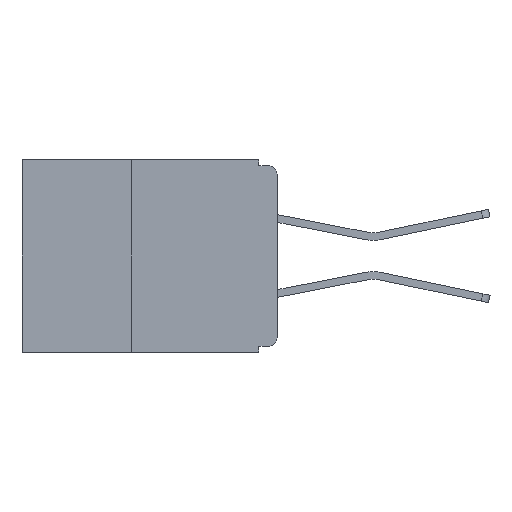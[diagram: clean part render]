
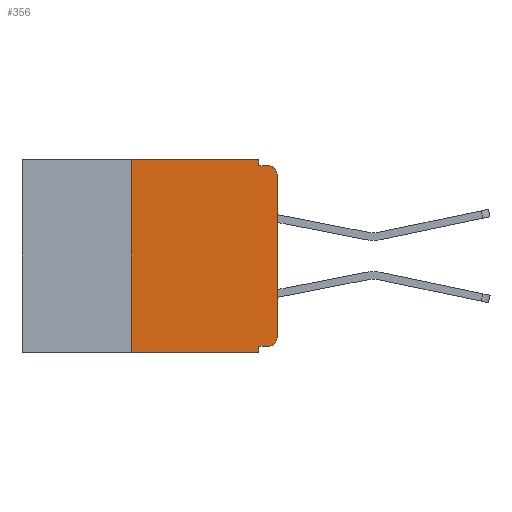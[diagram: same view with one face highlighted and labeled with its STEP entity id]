
A CAD part, left-side view. The second image highlights one B-rep face of the part: STEP entity #356.
In plain terms, the highlighted planar face has unit normal (-1, 0, 0).
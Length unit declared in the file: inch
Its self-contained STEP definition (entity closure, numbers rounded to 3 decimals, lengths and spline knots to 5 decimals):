
#95 = DIRECTION ( 'NONE',  ( 1., 0., 0. ) ) ;
#102 = DIRECTION ( 'NONE',  ( 0., 0., 1. ) ) ;
#113 = LINE ( 'NONE', #15190, #7937 ) ;
#356 = ADVANCED_FACE ( 'NONE', ( #10847 ), #14837, .F. ) ;
#819 = ORIENTED_EDGE ( 'NONE', *, *, #11171, .T. ) ;
#977 = CARTESIAN_POINT ( 'NONE',  ( 0., 0.031, -0.32 ) ) ;
#2271 = VERTEX_POINT ( 'NONE', #977 ) ;
#2440 = ORIENTED_EDGE ( 'NONE', *, *, #7968, .F. ) ;
#2616 = LINE ( 'NONE', #19415, #6744 ) ;
#2695 = CARTESIAN_POINT ( 'NONE',  ( 0., 0.031, -0.33 ) ) ;
#2927 = DIRECTION ( 'NONE',  ( -1., 0., 0. ) ) ;
#2969 = ORIENTED_EDGE ( 'NONE', *, *, #9448, .T. ) ;
#3210 = CARTESIAN_POINT ( 'NONE',  ( 0., 0., -0.025 ) ) ;
#3247 = CARTESIAN_POINT ( 'NONE',  ( 0., 0., -0.01 ) ) ;
#3523 = VECTOR ( 'NONE', #102, 39.37008 ) ;
#3764 = VERTEX_POINT ( 'NONE', #5513 ) ;
#3935 = CARTESIAN_POINT ( 'NONE',  ( 0., 0.015, -0.01 ) ) ;
#3939 = DIRECTION ( 'NONE',  ( 0., -1., 0. ) ) ;
#4456 = VERTEX_POINT ( 'NONE', #14680 ) ;
#4615 = CIRCLE ( 'NONE', #9679, 0.015 ) ;
#4623 = DIRECTION ( 'NONE',  ( 0., 0., -1. ) ) ;
#4911 = ORIENTED_EDGE ( 'NONE', *, *, #19390, .F. ) ;
#5103 = VERTEX_POINT ( 'NONE', #3210 ) ;
#5513 = CARTESIAN_POINT ( 'NONE',  ( 0., 0.25, 0. ) ) ;
#6025 = ORIENTED_EDGE ( 'NONE', *, *, #6124, .F. ) ;
#6053 = LINE ( 'NONE', #13020, #13586 ) ;
#6124 = EDGE_CURVE ( 'NONE', #19385, #2271, #113, .T. ) ;
#6363 = DIRECTION ( 'NONE',  ( 0., -1., 0. ) ) ;
#6632 = VERTEX_POINT ( 'NONE', #17980 ) ;
#6694 = VERTEX_POINT ( 'NONE', #13563 ) ;
#6744 = VECTOR ( 'NONE', #8948, 39.37008 ) ;
#6959 = ORIENTED_EDGE ( 'NONE', *, *, #15886, .T. ) ;
#7269 = DIRECTION ( 'NONE',  ( -1., 0., 0. ) ) ;
#7545 = ORIENTED_EDGE ( 'NONE', *, *, #10660, .T. ) ;
#7714 = CARTESIAN_POINT ( 'NONE',  ( 0., 0.015, -0.32 ) ) ;
#7893 = CARTESIAN_POINT ( 'NONE',  ( 0., 0.25, -0.33 ) ) ;
#7937 = VECTOR ( 'NONE', #9235, 39.37008 ) ;
#7946 = AXIS2_PLACEMENT_3D ( 'NONE', #15397, #95, #14928 ) ;
#7968 = EDGE_CURVE ( 'NONE', #16937, #15646, #19126, .T. ) ;
#8874 = CARTESIAN_POINT ( 'NONE',  ( 0., 0.031, -0.01 ) ) ;
#8948 = DIRECTION ( 'NONE',  ( 0., 0., 1. ) ) ;
#9162 = DIRECTION ( 'NONE',  ( 0., 0., -1. ) ) ;
#9235 = DIRECTION ( 'NONE',  ( 0., 1., 0. ) ) ;
#9357 = EDGE_CURVE ( 'NONE', #3764, #6694, #6053, .T. ) ;
#9448 = EDGE_CURVE ( 'NONE', #19385, #4456, #4615, .T. ) ;
#9679 = AXIS2_PLACEMENT_3D ( 'NONE', #12029, #2927, #13553 ) ;
#10184 = VECTOR ( 'NONE', #12079, 39.37008 ) ;
#10660 = EDGE_CURVE ( 'NONE', #4456, #5103, #2616, .T. ) ;
#10847 = FACE_OUTER_BOUND ( 'NONE', #15911, .T. ) ;
#11048 = ORIENTED_EDGE ( 'NONE', *, *, #17585, .F. ) ;
#11171 = EDGE_CURVE ( 'NONE', #5103, #15646, #12340, .T. ) ;
#12029 = CARTESIAN_POINT ( 'NONE',  ( 0., 0.015, -0.305 ) ) ;
#12079 = DIRECTION ( 'NONE',  ( 0., -1., 0. ) ) ;
#12302 = EDGE_CURVE ( 'NONE', #6632, #3764, #19590, .T. ) ;
#12340 = CIRCLE ( 'NONE', #17484, 0.015 ) ;
#13020 = CARTESIAN_POINT ( 'NONE',  ( 0., 0.437, 0. ) ) ;
#13553 = DIRECTION ( 'NONE',  ( 0., 0., -1. ) ) ;
#13563 = CARTESIAN_POINT ( 'NONE',  ( 0., 0.031, 0. ) ) ;
#13586 = VECTOR ( 'NONE', #3939, 39.37008 ) ;
#14056 = VECTOR ( 'NONE', #4623, 39.37008 ) ;
#14071 = ORIENTED_EDGE ( 'NONE', *, *, #12302, .F. ) ;
#14680 = CARTESIAN_POINT ( 'NONE',  ( 0., 0., -0.305 ) ) ;
#14837 = PLANE ( 'NONE',  #7946 ) ;
#14928 = DIRECTION ( 'NONE',  ( 0., 0., -1. ) ) ;
#15075 = CARTESIAN_POINT ( 'NONE',  ( 0., 0.437, -0.33 ) ) ;
#15143 = ORIENTED_EDGE ( 'NONE', *, *, #9357, .F. ) ;
#15190 = CARTESIAN_POINT ( 'NONE',  ( 0., 0., -0.32 ) ) ;
#15397 = CARTESIAN_POINT ( 'NONE',  ( 0., 0.437, 0. ) ) ;
#15631 = VECTOR ( 'NONE', #6363, 39.37008 ) ;
#15646 = VERTEX_POINT ( 'NONE', #3935 ) ;
#15886 = EDGE_CURVE ( 'NONE', #6632, #16304, #18649, .T. ) ;
#15911 = EDGE_LOOP ( 'NONE', ( #7545, #819, #2440, #11048, #15143, #14071, #6959, #4911, #6025, #2969 ) ) ;
#16231 = VECTOR ( 'NONE', #9162, 39.37008 ) ;
#16276 = CARTESIAN_POINT ( 'NONE',  ( 0., 0.015, -0.025 ) ) ;
#16304 = VERTEX_POINT ( 'NONE', #2695 ) ;
#16711 = CARTESIAN_POINT ( 'NONE',  ( 0., 0.031, -0.33 ) ) ;
#16937 = VERTEX_POINT ( 'NONE', #8874 ) ;
#17484 = AXIS2_PLACEMENT_3D ( 'NONE', #16276, #7269, #17772 ) ;
#17585 = EDGE_CURVE ( 'NONE', #6694, #16937, #19249, .T. ) ;
#17772 = DIRECTION ( 'NONE',  ( 0., 0., -1. ) ) ;
#17980 = CARTESIAN_POINT ( 'NONE',  ( 0., 0.25, -0.33 ) ) ;
#18051 = LINE ( 'NONE', #16711, #14056 ) ;
#18135 = CARTESIAN_POINT ( 'NONE',  ( 0., 0.031, 0. ) ) ;
#18649 = LINE ( 'NONE', #15075, #10184 ) ;
#19126 = LINE ( 'NONE', #3247, #15631 ) ;
#19249 = LINE ( 'NONE', #18135, #16231 ) ;
#19385 = VERTEX_POINT ( 'NONE', #7714 ) ;
#19390 = EDGE_CURVE ( 'NONE', #2271, #16304, #18051, .T. ) ;
#19415 = CARTESIAN_POINT ( 'NONE',  ( 0., 0., 0. ) ) ;
#19590 = LINE ( 'NONE', #7893, #3523 ) ;
